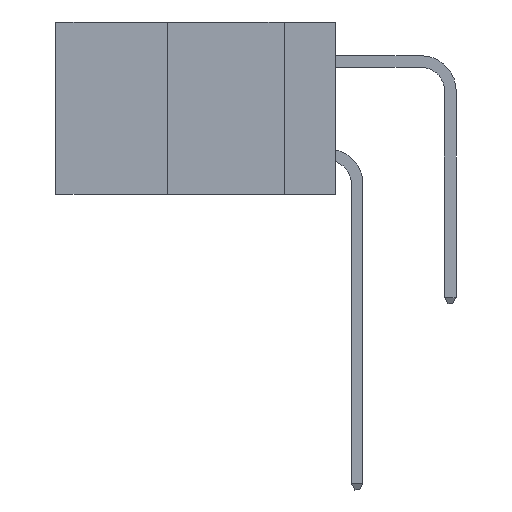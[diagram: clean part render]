
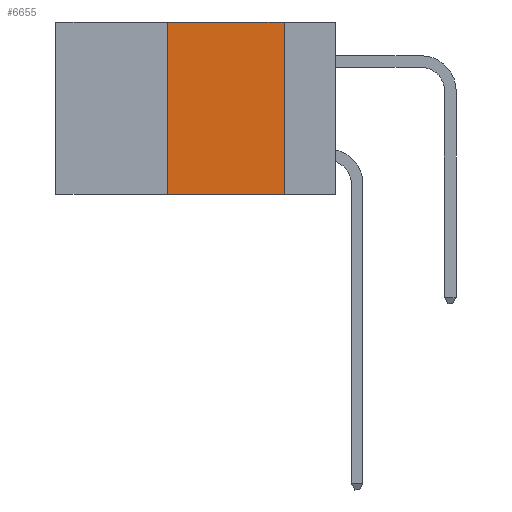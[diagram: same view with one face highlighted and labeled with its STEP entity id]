
A CAD part, left-side view. The second image highlights one B-rep face of the part: STEP entity #6655.
In plain terms, the highlighted planar face has unit normal (-1, 0, 0).
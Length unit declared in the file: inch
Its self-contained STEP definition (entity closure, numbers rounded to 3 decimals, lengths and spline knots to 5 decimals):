
#2084 = LINE ( 'NONE', #10723, #21209 ) ;
#4412 = ORIENTED_EDGE ( 'NONE', *, *, #9466, .F. ) ;
#5710 = CARTESIAN_POINT ( 'NONE',  ( 0., 0.11, -0.37 ) ) ;
#6655 = ADVANCED_FACE ( 'NONE', ( #9513 ), #8333, .F. ) ;
#6873 = EDGE_CURVE ( 'NONE', #20989, #11811, #11625, .T. ) ;
#7424 = LINE ( 'NONE', #11894, #9472 ) ;
#8333 = PLANE ( 'NONE',  #19627 ) ;
#8365 = CARTESIAN_POINT ( 'NONE',  ( 0., 0.11, 0. ) ) ;
#8546 = DIRECTION ( 'NONE',  ( 0., -1., 0. ) ) ;
#9466 = EDGE_CURVE ( 'NONE', #16277, #23586, #14251, .T. ) ;
#9472 = VECTOR ( 'NONE', #9731, 39.37008 ) ;
#9501 = CARTESIAN_POINT ( 'NONE',  ( 0., 0.36, -0.37 ) ) ;
#9513 = FACE_OUTER_BOUND ( 'NONE', #20908, .T. ) ;
#9731 = DIRECTION ( 'NONE',  ( 0., -1., 0. ) ) ;
#10723 = CARTESIAN_POINT ( 'NONE',  ( 0., 0.6, -0.37 ) ) ;
#11370 = DIRECTION ( 'NONE',  ( 0., 0., -1. ) ) ;
#11625 = LINE ( 'NONE', #8365, #17681 ) ;
#11811 = VERTEX_POINT ( 'NONE', #5710 ) ;
#11894 = CARTESIAN_POINT ( 'NONE',  ( 0., 0.6, 0. ) ) ;
#14251 = LINE ( 'NONE', #21485, #25840 ) ;
#16277 = VERTEX_POINT ( 'NONE', #9501 ) ;
#17221 = DIRECTION ( 'NONE',  ( 1., 0., 0. ) ) ;
#17681 = VECTOR ( 'NONE', #11370, 39.37008 ) ;
#19267 = CARTESIAN_POINT ( 'NONE',  ( 0., 0.6, 0. ) ) ;
#19627 = AXIS2_PLACEMENT_3D ( 'NONE', #19267, #17221, #25917 ) ;
#19735 = DIRECTION ( 'NONE',  ( 0., 0., 1. ) ) ;
#20294 = CARTESIAN_POINT ( 'NONE',  ( 0., 0.11, 0. ) ) ;
#20908 = EDGE_LOOP ( 'NONE', ( #26698, #24502, #4412, #28087 ) ) ;
#20989 = VERTEX_POINT ( 'NONE', #20294 ) ;
#21209 = VECTOR ( 'NONE', #8546, 39.37008 ) ;
#21485 = CARTESIAN_POINT ( 'NONE',  ( 0., 0.36, 0. ) ) ;
#23330 = CARTESIAN_POINT ( 'NONE',  ( 0., 0.36, 0. ) ) ;
#23586 = VERTEX_POINT ( 'NONE', #23330 ) ;
#24502 = ORIENTED_EDGE ( 'NONE', *, *, #27154, .F. ) ;
#25840 = VECTOR ( 'NONE', #19735, 39.37008 ) ;
#25917 = DIRECTION ( 'NONE',  ( 0., 0., -1. ) ) ;
#25927 = EDGE_CURVE ( 'NONE', #16277, #11811, #2084, .T. ) ;
#26698 = ORIENTED_EDGE ( 'NONE', *, *, #6873, .F. ) ;
#27154 = EDGE_CURVE ( 'NONE', #23586, #20989, #7424, .T. ) ;
#28087 = ORIENTED_EDGE ( 'NONE', *, *, #25927, .T. ) ;
